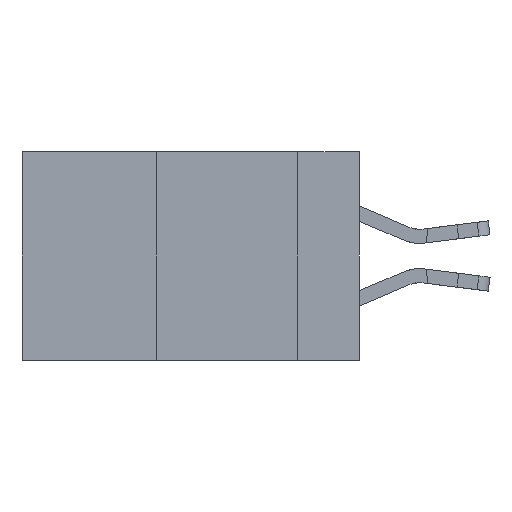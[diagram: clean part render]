
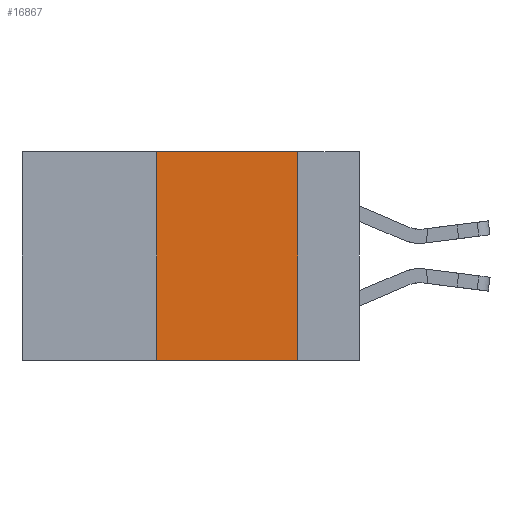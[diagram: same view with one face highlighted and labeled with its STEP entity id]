
A CAD part, left-side view. The second image highlights one B-rep face of the part: STEP entity #16867.
In plain terms, the highlighted planar face has unit normal (-1, 0, 0).
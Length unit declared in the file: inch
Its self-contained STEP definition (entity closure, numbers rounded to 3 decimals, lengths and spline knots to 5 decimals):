
#15 = CARTESIAN_POINT ( 'NONE',  ( 0., 0.36, -0.37 ) ) ;
#303 = PLANE ( 'NONE',  #1705 ) ;
#1452 = DIRECTION ( 'NONE',  ( 0., 0., -1. ) ) ;
#1502 = EDGE_CURVE ( 'NONE', #13013, #17503, #16295, .T. ) ;
#1606 = VECTOR ( 'NONE', #14149, 39.37008 ) ;
#1705 = AXIS2_PLACEMENT_3D ( 'NONE', #7193, #17146, #1452 ) ;
#1856 = CARTESIAN_POINT ( 'NONE',  ( 0., 0.11, 0. ) ) ;
#2794 = ORIENTED_EDGE ( 'NONE', *, *, #9999, .F. ) ;
#3361 = CARTESIAN_POINT ( 'NONE',  ( 0., 0.36, 0. ) ) ;
#4055 = VECTOR ( 'NONE', #17796, 39.37008 ) ;
#5407 = DIRECTION ( 'NONE',  ( 0., -1., 0. ) ) ;
#5575 = LINE ( 'NONE', #15455, #1606 ) ;
#5702 = EDGE_LOOP ( 'NONE', ( #14669, #13251, #2794, #6526 ) ) ;
#5753 = LINE ( 'NONE', #9315, #8657 ) ;
#6526 = ORIENTED_EDGE ( 'NONE', *, *, #8406, .T. ) ;
#7193 = CARTESIAN_POINT ( 'NONE',  ( 0., 0.6, 0. ) ) ;
#8084 = VECTOR ( 'NONE', #5407, 39.37008 ) ;
#8406 = EDGE_CURVE ( 'NONE', #11683, #16436, #15005, .T. ) ;
#8657 = VECTOR ( 'NONE', #12310, 39.37008 ) ;
#9315 = CARTESIAN_POINT ( 'NONE',  ( 0., 0.11, 0. ) ) ;
#9999 = EDGE_CURVE ( 'NONE', #11683, #13013, #5575, .T. ) ;
#11473 = EDGE_CURVE ( 'NONE', #17503, #16436, #5753, .T. ) ;
#11683 = VERTEX_POINT ( 'NONE', #15 ) ;
#12310 = DIRECTION ( 'NONE',  ( 0., 0., -1. ) ) ;
#12494 = CARTESIAN_POINT ( 'NONE',  ( 0., 0.6, -0.37 ) ) ;
#13013 = VERTEX_POINT ( 'NONE', #3361 ) ;
#13251 = ORIENTED_EDGE ( 'NONE', *, *, #1502, .F. ) ;
#13734 = CARTESIAN_POINT ( 'NONE',  ( 0., 0.6, 0. ) ) ;
#14149 = DIRECTION ( 'NONE',  ( 0., 0., 1. ) ) ;
#14669 = ORIENTED_EDGE ( 'NONE', *, *, #11473, .F. ) ;
#15005 = LINE ( 'NONE', #12494, #8084 ) ;
#15455 = CARTESIAN_POINT ( 'NONE',  ( 0., 0.36, 0. ) ) ;
#15870 = CARTESIAN_POINT ( 'NONE',  ( 0., 0.11, -0.37 ) ) ;
#16295 = LINE ( 'NONE', #13734, #4055 ) ;
#16436 = VERTEX_POINT ( 'NONE', #15870 ) ;
#16535 = FACE_OUTER_BOUND ( 'NONE', #5702, .T. ) ;
#16867 = ADVANCED_FACE ( 'NONE', ( #16535 ), #303, .F. ) ;
#17146 = DIRECTION ( 'NONE',  ( 1., 0., 0. ) ) ;
#17503 = VERTEX_POINT ( 'NONE', #1856 ) ;
#17796 = DIRECTION ( 'NONE',  ( 0., -1., 0. ) ) ;
